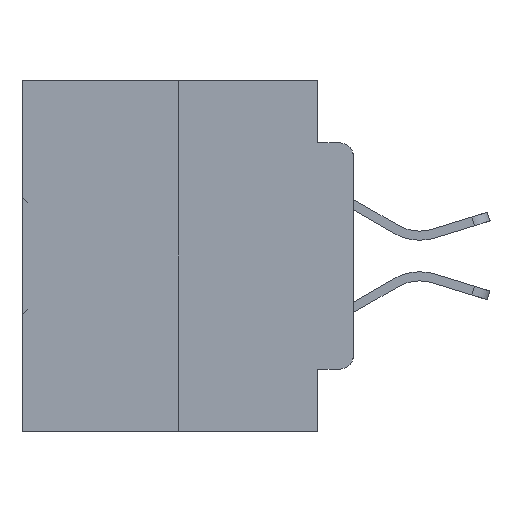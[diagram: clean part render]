
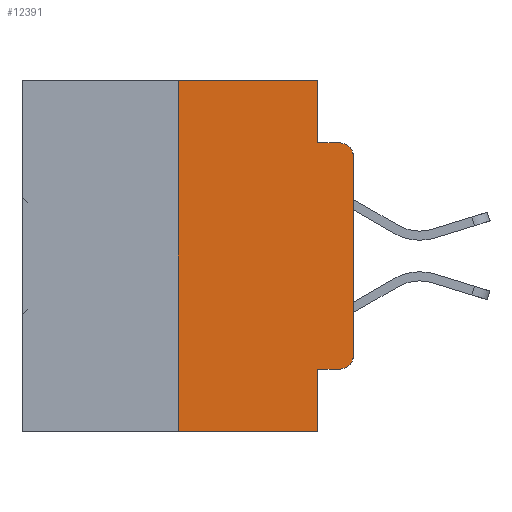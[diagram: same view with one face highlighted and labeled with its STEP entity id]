
A CAD part, left-side view. The second image highlights one B-rep face of the part: STEP entity #12391.
In plain terms, the highlighted planar face has unit normal (-1, 0, 0).
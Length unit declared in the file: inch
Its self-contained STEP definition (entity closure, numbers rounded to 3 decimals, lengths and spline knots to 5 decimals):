
#263 = ORIENTED_EDGE ( 'NONE', *, *, #27049, .T. ) ;
#321 = VERTEX_POINT ( 'NONE', #25469 ) ;
#566 = CARTESIAN_POINT ( 'NONE',  ( 0., 0.473, 0. ) ) ;
#615 = DIRECTION ( 'NONE',  ( 0., -1., 0. ) ) ;
#816 = CARTESIAN_POINT ( 'NONE',  ( 0., 0., 0. ) ) ;
#1216 = ORIENTED_EDGE ( 'NONE', *, *, #23432, .T. ) ;
#1306 = CARTESIAN_POINT ( 'NONE',  ( 0., 0.473, 0. ) ) ;
#1505 = VECTOR ( 'NONE', #30863, 39.37008 ) ;
#1686 = VECTOR ( 'NONE', #615, 39.37008 ) ;
#1770 = DIRECTION ( 'NONE',  ( 0., 0., -1. ) ) ;
#1992 = EDGE_CURVE ( 'NONE', #17997, #29954, #18438, .T. ) ;
#2127 = VECTOR ( 'NONE', #13763, 39.37008 ) ;
#2214 = FACE_OUTER_BOUND ( 'NONE', #27873, .T. ) ;
#2912 = PLANE ( 'NONE',  #21477 ) ;
#3096 = EDGE_CURVE ( 'NONE', #21672, #27193, #14994, .T. ) ;
#3258 = DIRECTION ( 'NONE',  ( 1., 0., 0. ) ) ;
#3704 = CARTESIAN_POINT ( 'NONE',  ( 0., 0., -0.1085 ) ) ;
#3777 = CARTESIAN_POINT ( 'NONE',  ( 0., 0., -0.3915 ) ) ;
#4028 = DIRECTION ( 'NONE',  ( 0., 0., -1. ) ) ;
#4714 = DIRECTION ( 'NONE',  ( -1., 0., 0. ) ) ;
#4970 = DIRECTION ( 'NONE',  ( 0., 0., -1. ) ) ;
#5702 = DIRECTION ( 'NONE',  ( 0., -1., 0. ) ) ;
#5914 = LINE ( 'NONE', #24884, #2127 ) ;
#6155 = CARTESIAN_POINT ( 'NONE',  ( 0., 0.051, -0.0885 ) ) ;
#6156 = VECTOR ( 'NONE', #5702, 39.37008 ) ;
#6166 = CARTESIAN_POINT ( 'NONE',  ( 0., 0.051, -0.4115 ) ) ;
#6800 = LINE ( 'NONE', #24058, #8941 ) ;
#7407 = ORIENTED_EDGE ( 'NONE', *, *, #33322, .T. ) ;
#7556 = CARTESIAN_POINT ( 'NONE',  ( 0., 0.02, -0.3915 ) ) ;
#7887 = ORIENTED_EDGE ( 'NONE', *, *, #29664, .F. ) ;
#8287 = AXIS2_PLACEMENT_3D ( 'NONE', #30923, #25420, #4028 ) ;
#8320 = EDGE_CURVE ( 'NONE', #9556, #29451, #6800, .T. ) ;
#8941 = VECTOR ( 'NONE', #19482, 39.37008 ) ;
#9556 = VERTEX_POINT ( 'NONE', #30732 ) ;
#9727 = CARTESIAN_POINT ( 'NONE',  ( 0., 0.051, -0.5 ) ) ;
#10833 = DIRECTION ( 'NONE',  ( 0., 0., -1. ) ) ;
#10996 = CARTESIAN_POINT ( 'NONE',  ( 0., 0.02, -0.4115 ) ) ;
#11310 = VECTOR ( 'NONE', #4970, 39.37008 ) ;
#11613 = CARTESIAN_POINT ( 'NONE',  ( 0., 0.051, -0.0885 ) ) ;
#11929 = ORIENTED_EDGE ( 'NONE', *, *, #8320, .F. ) ;
#12391 = ADVANCED_FACE ( 'NONE', ( #2214 ), #2912, .F. ) ;
#12594 = VERTEX_POINT ( 'NONE', #9727 ) ;
#12634 = CARTESIAN_POINT ( 'NONE',  ( 0., 0.051, 0. ) ) ;
#12888 = LINE ( 'NONE', #816, #1505 ) ;
#13667 = CARTESIAN_POINT ( 'NONE',  ( 0., 0.051, 0. ) ) ;
#13698 = EDGE_CURVE ( 'NONE', #29954, #321, #16005, .T. ) ;
#13763 = DIRECTION ( 'NONE',  ( 0., -1., 0. ) ) ;
#14327 = ORIENTED_EDGE ( 'NONE', *, *, #13698, .F. ) ;
#14994 = CIRCLE ( 'NONE', #27129, 0.02 ) ;
#15798 = ORIENTED_EDGE ( 'NONE', *, *, #23092, .F. ) ;
#16005 = LINE ( 'NONE', #6155, #1686 ) ;
#16533 = CIRCLE ( 'NONE', #8287, 0.02 ) ;
#17997 = VERTEX_POINT ( 'NONE', #13667 ) ;
#18438 = LINE ( 'NONE', #12634, #11310 ) ;
#18937 = VERTEX_POINT ( 'NONE', #3704 ) ;
#19482 = DIRECTION ( 'NONE',  ( 0., 0., 1. ) ) ;
#20067 = ORIENTED_EDGE ( 'NONE', *, *, #1992, .F. ) ;
#20868 = VECTOR ( 'NONE', #26747, 39.37008 ) ;
#21477 = AXIS2_PLACEMENT_3D ( 'NONE', #566, #3258, #10833 ) ;
#21672 = VERTEX_POINT ( 'NONE', #10996 ) ;
#22362 = ORIENTED_EDGE ( 'NONE', *, *, #29387, .T. ) ;
#22792 = VERTEX_POINT ( 'NONE', #34287 ) ;
#23092 = EDGE_CURVE ( 'NONE', #29451, #17997, #34201, .T. ) ;
#23432 = EDGE_CURVE ( 'NONE', #18937, #321, #16533, .T. ) ;
#24058 = CARTESIAN_POINT ( 'NONE',  ( 0., 0.25, 0. ) ) ;
#24881 = ORIENTED_EDGE ( 'NONE', *, *, #3096, .T. ) ;
#24884 = CARTESIAN_POINT ( 'NONE',  ( 0., 0.473, -0.5 ) ) ;
#25154 = DIRECTION ( 'NONE',  ( 0., -1., 0. ) ) ;
#25420 = DIRECTION ( 'NONE',  ( -1., 0., 0. ) ) ;
#25469 = CARTESIAN_POINT ( 'NONE',  ( 0., 0.02, -0.0885 ) ) ;
#26747 = DIRECTION ( 'NONE',  ( 0., 0., -1. ) ) ;
#27049 = EDGE_CURVE ( 'NONE', #22792, #21672, #30481, .T. ) ;
#27129 = AXIS2_PLACEMENT_3D ( 'NONE', #7556, #4714, #1770 ) ;
#27193 = VERTEX_POINT ( 'NONE', #3777 ) ;
#27873 = EDGE_LOOP ( 'NONE', ( #22362, #1216, #14327, #20067, #15798, #11929, #7407, #7887, #263, #24881 ) ) ;
#27993 = LINE ( 'NONE', #29098, #20868 ) ;
#29098 = CARTESIAN_POINT ( 'NONE',  ( 0., 0.051, 0. ) ) ;
#29387 = EDGE_CURVE ( 'NONE', #27193, #18937, #12888, .T. ) ;
#29451 = VERTEX_POINT ( 'NONE', #30979 ) ;
#29664 = EDGE_CURVE ( 'NONE', #22792, #12594, #27993, .T. ) ;
#29954 = VERTEX_POINT ( 'NONE', #11613 ) ;
#30481 = LINE ( 'NONE', #6166, #6156 ) ;
#30732 = CARTESIAN_POINT ( 'NONE',  ( 0., 0.25, -0.5 ) ) ;
#30863 = DIRECTION ( 'NONE',  ( 0., 0., 1. ) ) ;
#30923 = CARTESIAN_POINT ( 'NONE',  ( 0., 0.02, -0.1085 ) ) ;
#30979 = CARTESIAN_POINT ( 'NONE',  ( 0., 0.25, 0. ) ) ;
#32927 = VECTOR ( 'NONE', #25154, 39.37008 ) ;
#33322 = EDGE_CURVE ( 'NONE', #9556, #12594, #5914, .T. ) ;
#34201 = LINE ( 'NONE', #1306, #32927 ) ;
#34287 = CARTESIAN_POINT ( 'NONE',  ( 0., 0.051, -0.4115 ) ) ;
